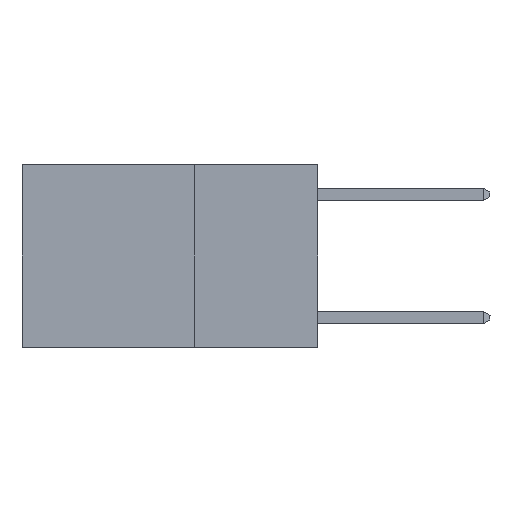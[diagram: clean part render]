
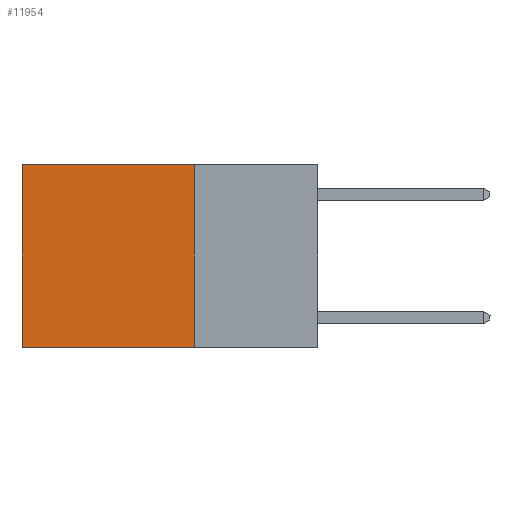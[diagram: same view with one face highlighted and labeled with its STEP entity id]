
A CAD part, left-side view. The second image highlights one B-rep face of the part: STEP entity #11954.
In plain terms, the highlighted planar face has unit normal (-1, 0, 0).
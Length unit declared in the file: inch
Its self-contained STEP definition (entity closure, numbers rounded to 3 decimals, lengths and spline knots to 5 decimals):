
#155 = CARTESIAN_POINT ( 'NONE',  ( 0.2625, 0.25, -0.37 ) ) ;
#995 = PLANE ( 'NONE',  #7421 ) ;
#1174 = LINE ( 'NONE', #3047, #17022 ) ;
#2070 = CARTESIAN_POINT ( 'NONE',  ( 0.2625, 0.6, -0.37 ) ) ;
#2296 = VERTEX_POINT ( 'NONE', #2070 ) ;
#2313 = EDGE_CURVE ( 'NONE', #6322, #2296, #13550, .T. ) ;
#3047 = CARTESIAN_POINT ( 'NONE',  ( 0.2625, 0.25, 0. ) ) ;
#3590 = DIRECTION ( 'NONE',  ( 0., 1., 0. ) ) ;
#5271 = VECTOR ( 'NONE', #17653, 39.37008 ) ;
#5389 = CARTESIAN_POINT ( 'NONE',  ( 0.2625, 0.6, 0. ) ) ;
#5789 = VECTOR ( 'NONE', #3590, 39.37008 ) ;
#6208 = FACE_OUTER_BOUND ( 'NONE', #6852, .T. ) ;
#6322 = VERTEX_POINT ( 'NONE', #155 ) ;
#6852 = EDGE_LOOP ( 'NONE', ( #7514, #7671, #7773, #7879 ) ) ;
#7174 = DIRECTION ( 'NONE',  ( 0., 0., -1. ) ) ;
#7421 = AXIS2_PLACEMENT_3D ( 'NONE', #10238, #16369, #7174 ) ;
#7514 = ORIENTED_EDGE ( 'NONE', *, *, #17728, .T. ) ;
#7535 = CARTESIAN_POINT ( 'NONE',  ( 0.2625, 0.25, 0. ) ) ;
#7671 = ORIENTED_EDGE ( 'NONE', *, *, #2313, .F. ) ;
#7773 = ORIENTED_EDGE ( 'NONE', *, *, #18757, .F. ) ;
#7879 = ORIENTED_EDGE ( 'NONE', *, *, #7985, .T. ) ;
#7985 = EDGE_CURVE ( 'NONE', #8859, #9043, #14802, .T. ) ;
#8276 = CARTESIAN_POINT ( 'NONE',  ( 0.2625, 0.6, 0. ) ) ;
#8859 = VERTEX_POINT ( 'NONE', #13860 ) ;
#9043 = VERTEX_POINT ( 'NONE', #8276 ) ;
#9091 = DIRECTION ( 'NONE',  ( 0., 1., 0. ) ) ;
#9256 = DIRECTION ( 'NONE',  ( 0., 0., -1. ) ) ;
#10238 = CARTESIAN_POINT ( 'NONE',  ( 0.2625, 0.25, 0. ) ) ;
#11954 = ADVANCED_FACE ( 'NONE', ( #6208 ), #995, .F. ) ;
#13550 = LINE ( 'NONE', #14397, #5789 ) ;
#13860 = CARTESIAN_POINT ( 'NONE',  ( 0.2625, 0.25, 0. ) ) ;
#14397 = CARTESIAN_POINT ( 'NONE',  ( 0.2625, 0.25, -0.37 ) ) ;
#14802 = LINE ( 'NONE', #7535, #18322 ) ;
#16369 = DIRECTION ( 'NONE',  ( 1., 0., 0. ) ) ;
#17022 = VECTOR ( 'NONE', #9256, 39.37008 ) ;
#17510 = LINE ( 'NONE', #5389, #5271 ) ;
#17653 = DIRECTION ( 'NONE',  ( 0., 0., -1. ) ) ;
#17728 = EDGE_CURVE ( 'NONE', #9043, #2296, #17510, .T. ) ;
#18322 = VECTOR ( 'NONE', #9091, 39.37008 ) ;
#18757 = EDGE_CURVE ( 'NONE', #8859, #6322, #1174, .T. ) ;
